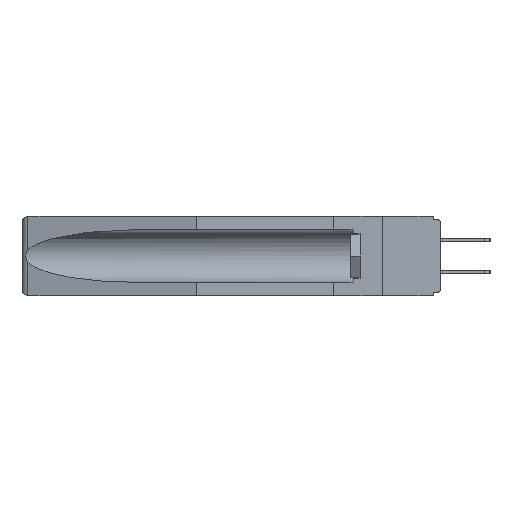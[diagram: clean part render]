
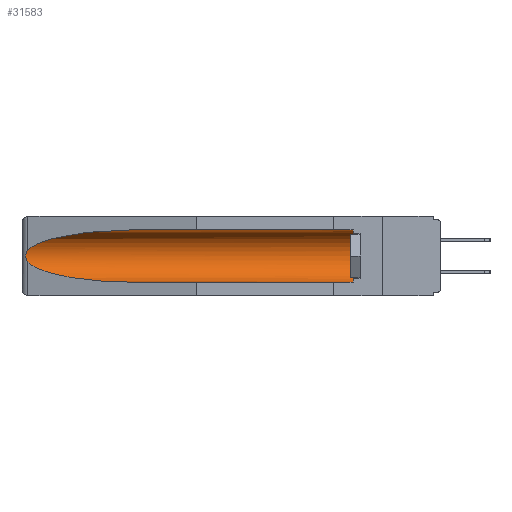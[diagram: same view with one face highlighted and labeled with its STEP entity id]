
A CAD part, left-side view. The second image highlights one B-rep face of the part: STEP entity #31583.
In plain terms, the highlighted cylindrical face has radius 2.857 mm (diameter 5.715 mm), a partial arc.
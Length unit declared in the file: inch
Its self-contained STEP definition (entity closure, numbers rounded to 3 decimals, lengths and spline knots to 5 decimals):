
#1712 = CARTESIAN_POINT ( 'NONE',  ( 0.155, 0.126, -0.284 ) ) ;
#2100 = EDGE_CURVE ( 'NONE', #19395, #33213, #7429, .T. ) ;
#2111 = CARTESIAN_POINT ( 'NONE',  ( 0.2675, 1.53308, -0.16763 ) ) ;
#2910 = LINE ( 'NONE', #27937, #8128 ) ;
#3639 = VECTOR ( 'NONE', #8484, 39.37008 ) ;
#4018 = ORIENTED_EDGE ( 'NONE', *, *, #2100, .T. ) ;
#4506 = CARTESIAN_POINT ( 'NONE',  ( 0.155, -0.30754, -0.1715 ) ) ;
#4959 = AXIS2_PLACEMENT_3D ( 'NONE', #4506, #12262, #24892 ) ;
#6801 = EDGE_LOOP ( 'NONE', ( #19783, #10386, #12817, #21128, #4018, #29358 ) ) ;
#6843 = CARTESIAN_POINT ( 'NONE',  ( 0.26654, 1.53092, -0.15636 ) ) ;
#7355 = CARTESIAN_POINT ( 'NONE',  ( 0.155, 0.126, -0.059 ) ) ;
#7429 = CIRCLE ( 'NONE', #17594, 0.1125 ) ;
#8128 = VECTOR ( 'NONE', #30589, 39.37008 ) ;
#8484 = DIRECTION ( 'NONE',  ( 0., 1., 0. ) ) ;
#8764 = EDGE_CURVE ( 'NONE', #19395, #20092, #2910, .T. ) ;
#9695 = CARTESIAN_POINT ( 'NONE',  ( 0.26537, 1.52718, -0.19328 ) ) ;
#9866 = CARTESIAN_POINT ( 'NONE',  ( 0.26537, 1.52718, -0.19328 ) ) ;
#10386 = ORIENTED_EDGE ( 'NONE', *, *, #15317, .T. ) ;
#10740 = CARTESIAN_POINT ( 'NONE',  ( 0.25451, 1.48313, -0.09465 ) ) ;
#10865 = CARTESIAN_POINT ( 'NONE',  ( 0.21114, 1.30732, -0.059 ) ) ;
#12237 = CARTESIAN_POINT ( 'NONE',  ( 0.155, 1.07973, -0.059 ) ) ;
#12262 = DIRECTION ( 'NONE',  ( 0., 1., 0. ) ) ;
#12817 = ORIENTED_EDGE ( 'NONE', *, *, #19512, .T. ) ;
#13163 = B_SPLINE_CURVE_WITH_KNOTS ( 'NONE', 3,
 ( #32620, #19808, #6843, #14696, #2111, #27507, #22617, #19694, #32825, #9866 ),
 .UNSPECIFIED., .F., .F.,
 ( 4, 2, 2, 2, 4 ),
 ( 0., 0.00029, 0.00058, 0.00087, 0.00117 ),
 .UNSPECIFIED. ) ;
#13956 = CARTESIAN_POINT ( 'NONE',  ( 0.26537, 1.52718, -0.14972 ) ) ;
#14095 = CARTESIAN_POINT ( 'NONE',  ( 0.155, 0.126, -0.1715 ) ) ;
#14293 = VERTEX_POINT ( 'NONE', #12237 ) ;
#14696 = CARTESIAN_POINT ( 'NONE',  ( 0.2673, 1.5327, -0.16383 ) ) ;
#14853 = CARTESIAN_POINT ( 'NONE',  ( 0.21114, 1.30732, -0.284 ) ) ;
#15317 = EDGE_CURVE ( 'NONE', #29965, #29168, #13163, .T. ) ;
#16473 = CARTESIAN_POINT ( 'NONE',  ( 0.155, -0.30754, -0.059 ) ) ;
#17104 =( BOUNDED_CURVE ( )  B_SPLINE_CURVE ( 3, ( #9695, #30324, #14853, #20282 ),
 .UNSPECIFIED., .F., .F. ) 
 B_SPLINE_CURVE_WITH_KNOTS ( ( 4, 4 ),
 ( 0.1948, 1.5708 ),
 .UNSPECIFIED. ) 
 CURVE ( )  GEOMETRIC_REPRESENTATION_ITEM ( )  RATIONAL_B_SPLINE_CURVE ( ( 1., 0.848, 0.848, 1. ) ) 
 REPRESENTATION_ITEM ( '' )  );
#17378 = CARTESIAN_POINT ( 'NONE',  ( 0.26537, 1.52718, -0.19328 ) ) ;
#17594 = AXIS2_PLACEMENT_3D ( 'NONE', #14095, #19304, #21885 ) ;
#18844 = CYLINDRICAL_SURFACE ( 'NONE', #4959, 0.1125 ) ;
#19304 = DIRECTION ( 'NONE',  ( 0., -1., 0. ) ) ;
#19395 = VERTEX_POINT ( 'NONE', #1712 ) ;
#19512 = EDGE_CURVE ( 'NONE', #29168, #20092, #17104, .T. ) ;
#19694 = CARTESIAN_POINT ( 'NONE',  ( 0.26655, 1.53094, -0.18657 ) ) ;
#19783 = ORIENTED_EDGE ( 'NONE', *, *, #31682, .T. ) ;
#19808 = CARTESIAN_POINT ( 'NONE',  ( 0.26597, 1.52961, -0.15275 ) ) ;
#20053 = CARTESIAN_POINT ( 'NONE',  ( 0.155, 1.07973, -0.284 ) ) ;
#20092 = VERTEX_POINT ( 'NONE', #20053 ) ;
#20224 =( BOUNDED_CURVE ( )  B_SPLINE_CURVE ( 3, ( #26338, #10865, #10740, #31487 ),
 .UNSPECIFIED., .F., .F. ) 
 B_SPLINE_CURVE_WITH_KNOTS ( ( 4, 4 ),
 ( 4.71239, 6.08839 ),
 .UNSPECIFIED. ) 
 CURVE ( )  GEOMETRIC_REPRESENTATION_ITEM ( )  RATIONAL_B_SPLINE_CURVE ( ( 1., 0.848, 0.848, 1. ) ) 
 REPRESENTATION_ITEM ( '' )  );
#20282 = CARTESIAN_POINT ( 'NONE',  ( 0.155, 1.07973, -0.284 ) ) ;
#21128 = ORIENTED_EDGE ( 'NONE', *, *, #8764, .F. ) ;
#21885 = DIRECTION ( 'NONE',  ( 0., 0., 1. ) ) ;
#22617 = CARTESIAN_POINT ( 'NONE',  ( 0.2673, 1.53269, -0.17917 ) ) ;
#23669 = FACE_OUTER_BOUND ( 'NONE', #6801, .T. ) ;
#24179 = LINE ( 'NONE', #16473, #3639 ) ;
#24892 = DIRECTION ( 'NONE',  ( 0., 0., 1. ) ) ;
#25925 = EDGE_CURVE ( 'NONE', #33213, #14293, #24179, .T. ) ;
#26338 = CARTESIAN_POINT ( 'NONE',  ( 0.155, 1.07973, -0.059 ) ) ;
#27507 = CARTESIAN_POINT ( 'NONE',  ( 0.2675, 1.53308, -0.17534 ) ) ;
#27937 = CARTESIAN_POINT ( 'NONE',  ( 0.155, -0.30754, -0.284 ) ) ;
#29168 = VERTEX_POINT ( 'NONE', #17378 ) ;
#29358 = ORIENTED_EDGE ( 'NONE', *, *, #25925, .T. ) ;
#29965 = VERTEX_POINT ( 'NONE', #13956 ) ;
#30324 = CARTESIAN_POINT ( 'NONE',  ( 0.25451, 1.48313, -0.24835 ) ) ;
#30589 = DIRECTION ( 'NONE',  ( 0., 1., 0. ) ) ;
#31487 = CARTESIAN_POINT ( 'NONE',  ( 0.26537, 1.52718, -0.14972 ) ) ;
#31583 = ADVANCED_FACE ( 'NONE', ( #23669 ), #18844, .F. ) ;
#31682 = EDGE_CURVE ( 'NONE', #14293, #29965, #20224, .T. ) ;
#32620 = CARTESIAN_POINT ( 'NONE',  ( 0.26537, 1.52718, -0.14972 ) ) ;
#32825 = CARTESIAN_POINT ( 'NONE',  ( 0.26597, 1.5296, -0.19026 ) ) ;
#33213 = VERTEX_POINT ( 'NONE', #7355 ) ;
